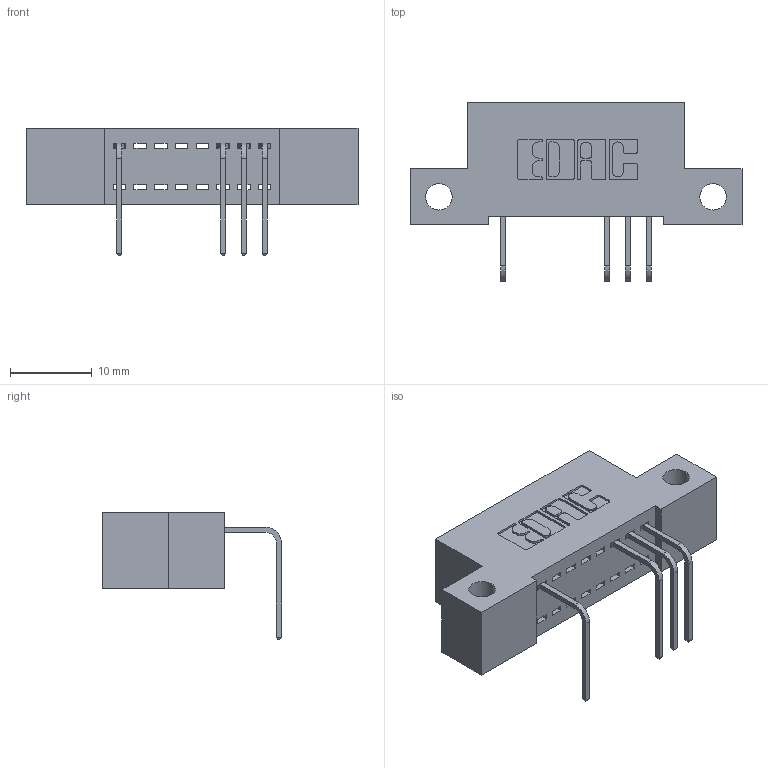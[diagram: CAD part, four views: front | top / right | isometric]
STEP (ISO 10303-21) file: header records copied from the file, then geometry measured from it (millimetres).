
FILE_DESCRIPTION (( 'STEP AP203' ), '1' );
FILE_NAME ('342-008-558-112.STEP', '2018-08-10T12:34:39', ( '' ), ( '' ), 'SwSTEP 2.0', 'SolidWorks 2016', '' );
FILE_SCHEMA (( 'CONFIG_CONTROL_DESIGN' ));
Length unit declared in the file: inch
Products named in the file (3): 342-008-558-112; 342 Part_Side Mount; 345-292-001_558 Tail - 2
Assembly tree (5 placements, depth 2):
  342-008-558-112
    342 Part_Side Mount
    345-292-001_558 Tail - 2  x4
Bounding box: 40.64 x 21.91 x 15.62 mm (x, y, z)
Volume: 3331.7 mm3; surface area: 3933.2 mm2
Topology: 5 solids, 5 shells, 398 faces, 1195 edges, 790 vertices
Faces by surface type: plane 290, cylinder 108
Entity records: 9115 total; most frequent: CARTESIAN_POINT 1602, ORIENTED_EDGE 1550, DIRECTION 1415, EDGE_CURVE 775, VECTOR 647, LINE 647, VERTEX_POINT 514, AXIS2_PLACEMENT_3D 384
